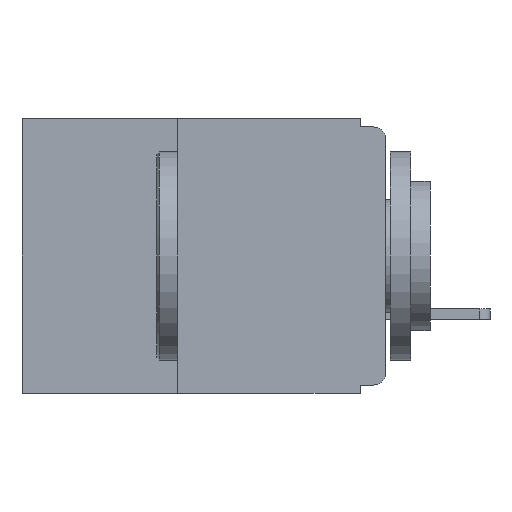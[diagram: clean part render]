
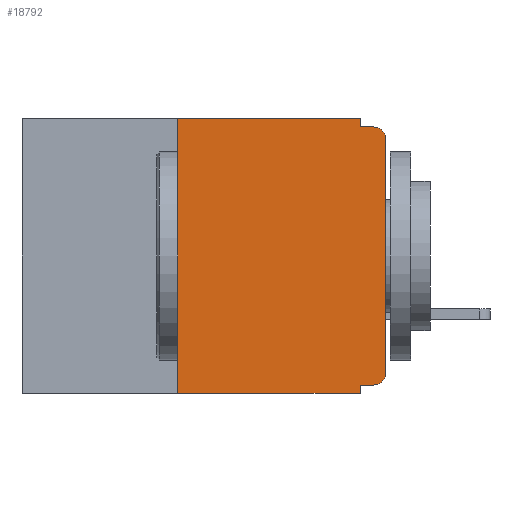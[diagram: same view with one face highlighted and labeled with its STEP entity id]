
A CAD part, left-side view. The second image highlights one B-rep face of the part: STEP entity #18792.
In plain terms, the highlighted planar face has unit normal (-1, 0, 0).
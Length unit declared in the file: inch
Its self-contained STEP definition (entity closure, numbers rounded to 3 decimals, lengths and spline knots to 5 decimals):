
#40 = DIRECTION ( 'NONE',  ( -1., 0., 0. ) ) ;
#548 = VECTOR ( 'NONE', #12373, 39.37008 ) ;
#849 = LINE ( 'NONE', #12465, #8354 ) ;
#1016 = LINE ( 'NONE', #6108, #548 ) ;
#1202 = ORIENTED_EDGE ( 'NONE', *, *, #15193, .T. ) ;
#1279 = CARTESIAN_POINT ( 'NONE',  ( 0., 0.25, 0. ) ) ;
#1694 = EDGE_CURVE ( 'NONE', #2379, #6051, #15682, .T. ) ;
#1891 = EDGE_CURVE ( 'NONE', #6051, #15330, #1016, .T. ) ;
#2379 = VERTEX_POINT ( 'NONE', #14510 ) ;
#2442 = LINE ( 'NONE', #6684, #9995 ) ;
#2551 = CARTESIAN_POINT ( 'NONE',  ( 0., 0.031, -0.33 ) ) ;
#2780 = LINE ( 'NONE', #10397, #14204 ) ;
#3815 = CARTESIAN_POINT ( 'NONE',  ( 0., 0.031, -0.01 ) ) ;
#4310 = PLANE ( 'NONE',  #10308 ) ;
#4585 = LINE ( 'NONE', #17131, #16475 ) ;
#4658 = EDGE_LOOP ( 'NONE', ( #1202, #5113, #13082, #13532, #17449, #13981, #17903, #7040, #11029, #18826 ) ) ;
#5027 = VERTEX_POINT ( 'NONE', #7493 ) ;
#5031 = EDGE_CURVE ( 'NONE', #2379, #5133, #18137, .T. ) ;
#5113 = ORIENTED_EDGE ( 'NONE', *, *, #17978, .T. ) ;
#5133 = VERTEX_POINT ( 'NONE', #6018 ) ;
#5870 = CIRCLE ( 'NONE', #15909, 0.015 ) ;
#6018 = CARTESIAN_POINT ( 'NONE',  ( 0., 0., -0.305 ) ) ;
#6051 = VERTEX_POINT ( 'NONE', #6546 ) ;
#6108 = CARTESIAN_POINT ( 'NONE',  ( 0., 0.031, -0.33 ) ) ;
#6546 = CARTESIAN_POINT ( 'NONE',  ( 0., 0.031, -0.32 ) ) ;
#6684 = CARTESIAN_POINT ( 'NONE',  ( 0., 0., 0. ) ) ;
#7022 = DIRECTION ( 'NONE',  ( 0., 0., -1. ) ) ;
#7040 = ORIENTED_EDGE ( 'NONE', *, *, #1891, .F. ) ;
#7056 = DIRECTION ( 'NONE',  ( -1., 0., 0. ) ) ;
#7081 = CARTESIAN_POINT ( 'NONE',  ( 0., 0.015, -0.305 ) ) ;
#7190 = LINE ( 'NONE', #18410, #18501 ) ;
#7361 = DIRECTION ( 'NONE',  ( 1., 0., 0. ) ) ;
#7466 = VERTEX_POINT ( 'NONE', #12440 ) ;
#7493 = CARTESIAN_POINT ( 'NONE',  ( 0., 0.25, -0.33 ) ) ;
#7541 = CARTESIAN_POINT ( 'NONE',  ( 0., 0., -0.01 ) ) ;
#7576 = EDGE_CURVE ( 'NONE', #5027, #11611, #4585, .T. ) ;
#8214 = CARTESIAN_POINT ( 'NONE',  ( 0., 0.015, -0.01 ) ) ;
#8308 = DIRECTION ( 'NONE',  ( 0., 0., 1. ) ) ;
#8354 = VECTOR ( 'NONE', #18306, 39.37008 ) ;
#9046 = CARTESIAN_POINT ( 'NONE',  ( 0., 0.015, -0.025 ) ) ;
#9641 = DIRECTION ( 'NONE',  ( 0., 0., -1. ) ) ;
#9995 = VECTOR ( 'NONE', #18520, 39.37008 ) ;
#10308 = AXIS2_PLACEMENT_3D ( 'NONE', #16229, #7361, #17686 ) ;
#10397 = CARTESIAN_POINT ( 'NONE',  ( 0., 0.437, -0.33 ) ) ;
#10539 = DIRECTION ( 'NONE',  ( 0., 0., -1. ) ) ;
#10643 = EDGE_CURVE ( 'NONE', #19172, #19126, #14216, .T. ) ;
#11029 = ORIENTED_EDGE ( 'NONE', *, *, #1694, .F. ) ;
#11198 = CARTESIAN_POINT ( 'NONE',  ( 0., 0.031, 0. ) ) ;
#11611 = VERTEX_POINT ( 'NONE', #1279 ) ;
#11781 = VECTOR ( 'NONE', #13799, 39.37008 ) ;
#12018 = DIRECTION ( 'NONE',  ( 0., -1., 0. ) ) ;
#12373 = DIRECTION ( 'NONE',  ( 0., 0., -1. ) ) ;
#12440 = CARTESIAN_POINT ( 'NONE',  ( 0., 0., -0.025 ) ) ;
#12465 = CARTESIAN_POINT ( 'NONE',  ( 0., 0.437, 0. ) ) ;
#13082 = ORIENTED_EDGE ( 'NONE', *, *, #10643, .F. ) ;
#13532 = ORIENTED_EDGE ( 'NONE', *, *, #14500, .F. ) ;
#13751 = VECTOR ( 'NONE', #12018, 39.37008 ) ;
#13799 = DIRECTION ( 'NONE',  ( 0., 1., 0. ) ) ;
#13981 = ORIENTED_EDGE ( 'NONE', *, *, #7576, .F. ) ;
#14204 = VECTOR ( 'NONE', #19143, 39.37008 ) ;
#14216 = LINE ( 'NONE', #7541, #13751 ) ;
#14500 = EDGE_CURVE ( 'NONE', #19128, #19172, #7190, .T. ) ;
#14510 = CARTESIAN_POINT ( 'NONE',  ( 0., 0.015, -0.32 ) ) ;
#14683 = FACE_OUTER_BOUND ( 'NONE', #4658, .T. ) ;
#15193 = EDGE_CURVE ( 'NONE', #5133, #7466, #2442, .T. ) ;
#15330 = VERTEX_POINT ( 'NONE', #2551 ) ;
#15682 = LINE ( 'NONE', #17430, #11781 ) ;
#15723 = EDGE_CURVE ( 'NONE', #11611, #19128, #849, .T. ) ;
#15909 = AXIS2_PLACEMENT_3D ( 'NONE', #9046, #40, #10539 ) ;
#16229 = CARTESIAN_POINT ( 'NONE',  ( 0., 0.437, 0. ) ) ;
#16357 = AXIS2_PLACEMENT_3D ( 'NONE', #7081, #7056, #7022 ) ;
#16475 = VECTOR ( 'NONE', #8308, 39.37008 ) ;
#17131 = CARTESIAN_POINT ( 'NONE',  ( 0., 0.25, -0.33 ) ) ;
#17430 = CARTESIAN_POINT ( 'NONE',  ( 0., 0., -0.32 ) ) ;
#17449 = ORIENTED_EDGE ( 'NONE', *, *, #15723, .F. ) ;
#17686 = DIRECTION ( 'NONE',  ( 0., 0., -1. ) ) ;
#17903 = ORIENTED_EDGE ( 'NONE', *, *, #18802, .T. ) ;
#17978 = EDGE_CURVE ( 'NONE', #7466, #19126, #5870, .T. ) ;
#18137 = CIRCLE ( 'NONE', #16357, 0.015 ) ;
#18306 = DIRECTION ( 'NONE',  ( 0., -1., 0. ) ) ;
#18410 = CARTESIAN_POINT ( 'NONE',  ( 0., 0.031, 0. ) ) ;
#18501 = VECTOR ( 'NONE', #9641, 39.37008 ) ;
#18520 = DIRECTION ( 'NONE',  ( 0., 0., 1. ) ) ;
#18792 = ADVANCED_FACE ( 'NONE', ( #14683 ), #4310, .F. ) ;
#18802 = EDGE_CURVE ( 'NONE', #5027, #15330, #2780, .T. ) ;
#18826 = ORIENTED_EDGE ( 'NONE', *, *, #5031, .T. ) ;
#19126 = VERTEX_POINT ( 'NONE', #8214 ) ;
#19128 = VERTEX_POINT ( 'NONE', #11198 ) ;
#19143 = DIRECTION ( 'NONE',  ( 0., -1., 0. ) ) ;
#19172 = VERTEX_POINT ( 'NONE', #3815 ) ;
